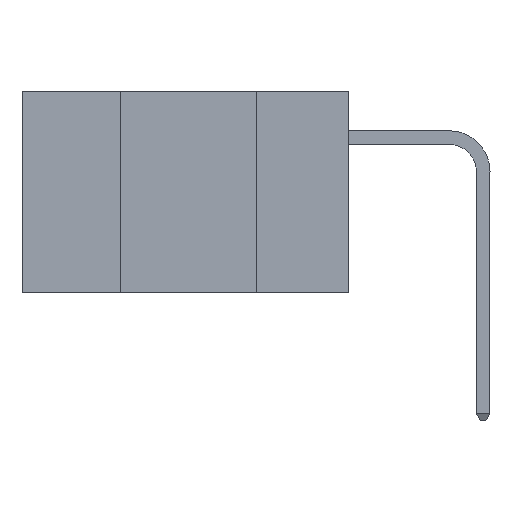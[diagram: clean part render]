
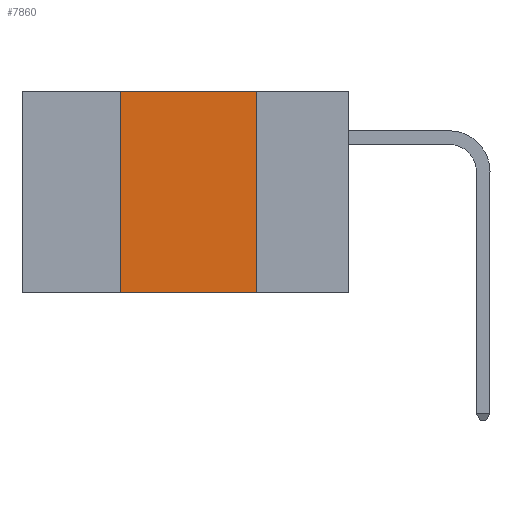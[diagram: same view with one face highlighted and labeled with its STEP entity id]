
A CAD part, left-side view. The second image highlights one B-rep face of the part: STEP entity #7860.
In plain terms, the highlighted planar face has unit normal (-1, 0, 0).
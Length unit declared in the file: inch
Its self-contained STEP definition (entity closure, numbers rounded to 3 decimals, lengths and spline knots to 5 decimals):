
#140 = VERTEX_POINT ( 'NONE', #4959 ) ;
#462 = AXIS2_PLACEMENT_3D ( 'NONE', #11429, #2145, #12388 ) ;
#1176 = DIRECTION ( 'NONE',  ( 0., 0., 1. ) ) ;
#1544 = EDGE_CURVE ( 'NONE', #12316, #5578, #5105, .T. ) ;
#1850 = ORIENTED_EDGE ( 'NONE', *, *, #12370, .T. ) ;
#2145 = DIRECTION ( 'NONE',  ( 1., 0., 0. ) ) ;
#2231 = VECTOR ( 'NONE', #4080, 39.37008 ) ;
#2312 = CARTESIAN_POINT ( 'NONE',  ( 0., 0.17, 0. ) ) ;
#2577 = EDGE_LOOP ( 'NONE', ( #12755, #10303, #5798, #1850 ) ) ;
#3026 = CARTESIAN_POINT ( 'NONE',  ( 0., 0.6, 0. ) ) ;
#4080 = DIRECTION ( 'NONE',  ( 0., -1., 0. ) ) ;
#4284 = CARTESIAN_POINT ( 'NONE',  ( 0., 0.42, 0. ) ) ;
#4306 = PLANE ( 'NONE',  #462 ) ;
#4959 = CARTESIAN_POINT ( 'NONE',  ( 0., 0.17, 0. ) ) ;
#5007 = VERTEX_POINT ( 'NONE', #10190 ) ;
#5105 = LINE ( 'NONE', #4284, #10172 ) ;
#5578 = VERTEX_POINT ( 'NONE', #11990 ) ;
#5702 = EDGE_CURVE ( 'NONE', #5578, #140, #10477, .T. ) ;
#5798 = ORIENTED_EDGE ( 'NONE', *, *, #1544, .F. ) ;
#5854 = CARTESIAN_POINT ( 'NONE',  ( 0., 0.42, -0.37 ) ) ;
#7860 = ADVANCED_FACE ( 'NONE', ( #8276 ), #4306, .F. ) ;
#7934 = CARTESIAN_POINT ( 'NONE',  ( 0., 0.6, -0.37 ) ) ;
#8276 = FACE_OUTER_BOUND ( 'NONE', #2577, .T. ) ;
#8532 = EDGE_CURVE ( 'NONE', #140, #5007, #12071, .T. ) ;
#9423 = VECTOR ( 'NONE', #10571, 39.37008 ) ;
#9946 = VECTOR ( 'NONE', #12866, 39.37008 ) ;
#10172 = VECTOR ( 'NONE', #1176, 39.37008 ) ;
#10190 = CARTESIAN_POINT ( 'NONE',  ( 0., 0.17, -0.37 ) ) ;
#10303 = ORIENTED_EDGE ( 'NONE', *, *, #5702, .F. ) ;
#10477 = LINE ( 'NONE', #3026, #2231 ) ;
#10571 = DIRECTION ( 'NONE',  ( 0., 0., -1. ) ) ;
#11429 = CARTESIAN_POINT ( 'NONE',  ( 0., 0.6, 0. ) ) ;
#11990 = CARTESIAN_POINT ( 'NONE',  ( 0., 0.42, 0. ) ) ;
#12071 = LINE ( 'NONE', #2312, #9423 ) ;
#12316 = VERTEX_POINT ( 'NONE', #5854 ) ;
#12370 = EDGE_CURVE ( 'NONE', #12316, #5007, #12558, .T. ) ;
#12388 = DIRECTION ( 'NONE',  ( 0., 0., -1. ) ) ;
#12558 = LINE ( 'NONE', #7934, #9946 ) ;
#12755 = ORIENTED_EDGE ( 'NONE', *, *, #8532, .F. ) ;
#12866 = DIRECTION ( 'NONE',  ( 0., -1., 0. ) ) ;
